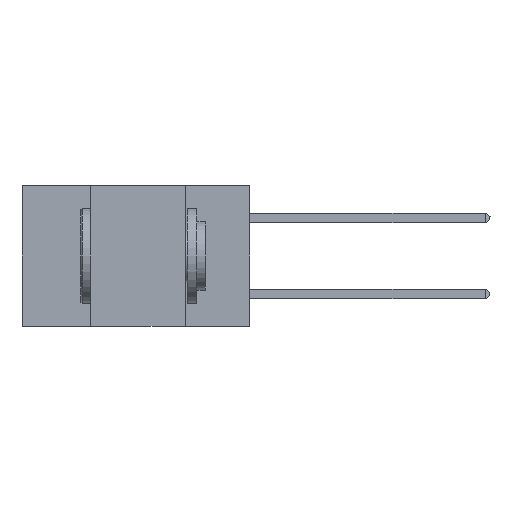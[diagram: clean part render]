
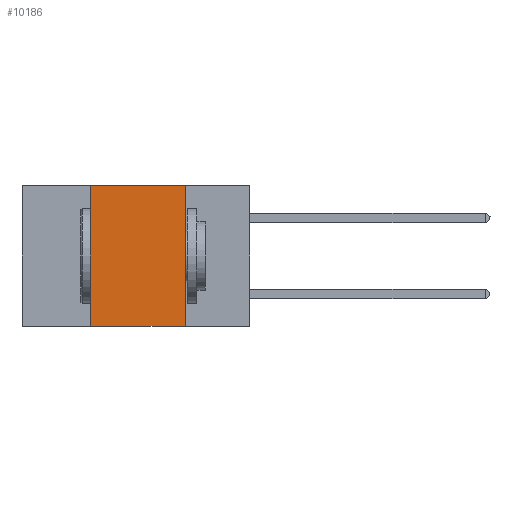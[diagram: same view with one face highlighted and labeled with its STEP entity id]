
A CAD part, left-side view. The second image highlights one B-rep face of the part: STEP entity #10186.
In plain terms, the highlighted planar face has unit normal (-1, 0, 0).
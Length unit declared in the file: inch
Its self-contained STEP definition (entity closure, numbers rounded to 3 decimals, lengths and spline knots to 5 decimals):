
#348 = DIRECTION ( 'NONE',  ( 1., 0., 0. ) ) ;
#433 = CARTESIAN_POINT ( 'NONE',  ( 0., 0.6, 0. ) ) ;
#676 = VERTEX_POINT ( 'NONE', #996 ) ;
#996 = CARTESIAN_POINT ( 'NONE',  ( 0., 0.17, 0. ) ) ;
#2021 = VERTEX_POINT ( 'NONE', #8563 ) ;
#2462 = DIRECTION ( 'NONE',  ( 0., 0., -1. ) ) ;
#2482 = VECTOR ( 'NONE', #11725, 39.37008 ) ;
#2530 = ORIENTED_EDGE ( 'NONE', *, *, #9069, .F. ) ;
#3150 = CARTESIAN_POINT ( 'NONE',  ( 0., 0.6, -0.37 ) ) ;
#3299 = LINE ( 'NONE', #10261, #11914 ) ;
#3527 = DIRECTION ( 'NONE',  ( 0., 0., -1. ) ) ;
#4030 = LINE ( 'NONE', #10517, #8573 ) ;
#4644 = ORIENTED_EDGE ( 'NONE', *, *, #6036, .T. ) ;
#4752 = VERTEX_POINT ( 'NONE', #5893 ) ;
#4840 = ORIENTED_EDGE ( 'NONE', *, *, #5045, .F. ) ;
#4966 = DIRECTION ( 'NONE',  ( 0., 0., 1. ) ) ;
#5045 = EDGE_CURVE ( 'NONE', #2021, #676, #3299, .T. ) ;
#5145 = LINE ( 'NONE', #3150, #2482 ) ;
#5448 = ORIENTED_EDGE ( 'NONE', *, *, #6977, .F. ) ;
#5893 = CARTESIAN_POINT ( 'NONE',  ( 0., 0.17, -0.37 ) ) ;
#6036 = EDGE_CURVE ( 'NONE', #11329, #4752, #5145, .T. ) ;
#6800 = AXIS2_PLACEMENT_3D ( 'NONE', #433, #348, #2462 ) ;
#6977 = EDGE_CURVE ( 'NONE', #676, #4752, #4030, .T. ) ;
#7708 = FACE_OUTER_BOUND ( 'NONE', #8037, .T. ) ;
#8037 = EDGE_LOOP ( 'NONE', ( #5448, #4840, #2530, #4644 ) ) ;
#8319 = CARTESIAN_POINT ( 'NONE',  ( 0., 0.42, 0. ) ) ;
#8374 = DIRECTION ( 'NONE',  ( 0., -1., 0. ) ) ;
#8563 = CARTESIAN_POINT ( 'NONE',  ( 0., 0.42, 0. ) ) ;
#8573 = VECTOR ( 'NONE', #3527, 39.37008 ) ;
#9069 = EDGE_CURVE ( 'NONE', #11329, #2021, #9294, .T. ) ;
#9294 = LINE ( 'NONE', #8319, #10681 ) ;
#9390 = PLANE ( 'NONE',  #6800 ) ;
#10186 = ADVANCED_FACE ( 'NONE', ( #7708 ), #9390, .F. ) ;
#10261 = CARTESIAN_POINT ( 'NONE',  ( 0., 0.6, 0. ) ) ;
#10517 = CARTESIAN_POINT ( 'NONE',  ( 0., 0.17, 0. ) ) ;
#10681 = VECTOR ( 'NONE', #4966, 39.37008 ) ;
#11329 = VERTEX_POINT ( 'NONE', #12579 ) ;
#11725 = DIRECTION ( 'NONE',  ( 0., -1., 0. ) ) ;
#11914 = VECTOR ( 'NONE', #8374, 39.37008 ) ;
#12579 = CARTESIAN_POINT ( 'NONE',  ( 0., 0.42, -0.37 ) ) ;
